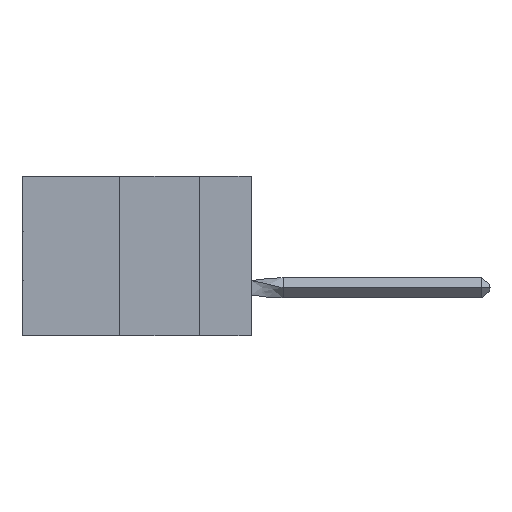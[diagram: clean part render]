
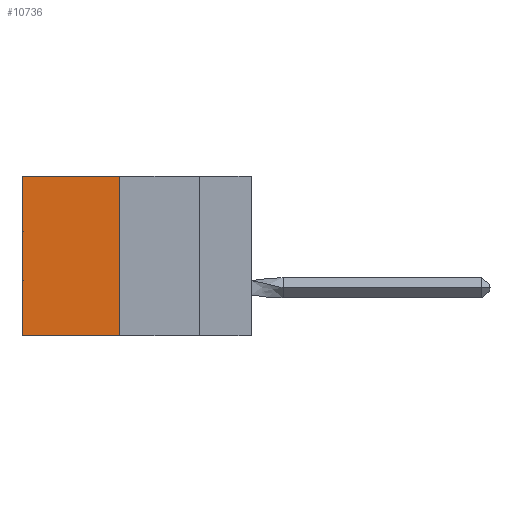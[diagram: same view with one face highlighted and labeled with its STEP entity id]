
A CAD part, left-side view. The second image highlights one B-rep face of the part: STEP entity #10736.
In plain terms, the highlighted planar face has unit normal (-1, 0, 0).
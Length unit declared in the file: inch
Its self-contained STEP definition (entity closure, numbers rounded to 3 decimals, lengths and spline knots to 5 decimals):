
#1268 = EDGE_LOOP ( 'NONE', ( #44782, #17903, #17036, #2817 ) ) ;
#1631 = AXIS2_PLACEMENT_3D ( 'NONE', #14071, #42016, #17612 ) ;
#2817 = ORIENTED_EDGE ( 'NONE', *, *, #4284, .T. ) ;
#3639 = CARTESIAN_POINT ( 'NONE',  ( 0.305, 0.413, 0. ) ) ;
#4284 = EDGE_CURVE ( 'NONE', #41292, #17914, #5164, .T. ) ;
#5164 = LINE ( 'NONE', #31909, #41944 ) ;
#7948 = VECTOR ( 'NONE', #34667, 39.37008 ) ;
#10032 = DIRECTION ( 'NONE',  ( 0., 0., -1. ) ) ;
#10210 = EDGE_CURVE ( 'NONE', #15788, #34587, #11222, .T. ) ;
#10614 = FACE_OUTER_BOUND ( 'NONE', #1268, .T. ) ;
#10736 = ADVANCED_FACE ( 'NONE', ( #10614 ), #31404, .F. ) ;
#11222 = LINE ( 'NONE', #31138, #7948 ) ;
#11750 = EDGE_CURVE ( 'NONE', #41292, #15788, #30357, .T. ) ;
#14071 = CARTESIAN_POINT ( 'NONE',  ( 0.305, 0.413, -0.5 ) ) ;
#15756 = VECTOR ( 'NONE', #18524, 39.37008 ) ;
#15788 = VERTEX_POINT ( 'NONE', #27751 ) ;
#16858 = CARTESIAN_POINT ( 'NONE',  ( 0.305, 0.72, -0.5 ) ) ;
#17036 = ORIENTED_EDGE ( 'NONE', *, *, #11750, .F. ) ;
#17612 = DIRECTION ( 'NONE',  ( 0., 0., -1. ) ) ;
#17626 = EDGE_CURVE ( 'NONE', #17914, #34587, #34394, .T. ) ;
#17903 = ORIENTED_EDGE ( 'NONE', *, *, #10210, .F. ) ;
#17914 = VERTEX_POINT ( 'NONE', #18613 ) ;
#18524 = DIRECTION ( 'NONE',  ( 0., 0., -1. ) ) ;
#18613 = CARTESIAN_POINT ( 'NONE',  ( 0.305, 0.72, 0. ) ) ;
#22329 = CARTESIAN_POINT ( 'NONE',  ( 0.305, 0.72, -0.5 ) ) ;
#23850 = CARTESIAN_POINT ( 'NONE',  ( 0.305, 0.413, -0.5 ) ) ;
#27751 = CARTESIAN_POINT ( 'NONE',  ( 0.305, 0.413, -0.5 ) ) ;
#28711 = VECTOR ( 'NONE', #10032, 39.37008 ) ;
#30357 = LINE ( 'NONE', #23850, #28711 ) ;
#31138 = CARTESIAN_POINT ( 'NONE',  ( 0.305, 0.413, -0.5 ) ) ;
#31404 = PLANE ( 'NONE',  #1631 ) ;
#31909 = CARTESIAN_POINT ( 'NONE',  ( 0.305, 0.413, 0. ) ) ;
#34394 = LINE ( 'NONE', #22329, #15756 ) ;
#34587 = VERTEX_POINT ( 'NONE', #16858 ) ;
#34667 = DIRECTION ( 'NONE',  ( 0., 1., 0. ) ) ;
#35429 = DIRECTION ( 'NONE',  ( 0., 1., 0. ) ) ;
#41292 = VERTEX_POINT ( 'NONE', #3639 ) ;
#41944 = VECTOR ( 'NONE', #35429, 39.37008 ) ;
#42016 = DIRECTION ( 'NONE',  ( 1., 0., 0. ) ) ;
#44782 = ORIENTED_EDGE ( 'NONE', *, *, #17626, .T. ) ;
